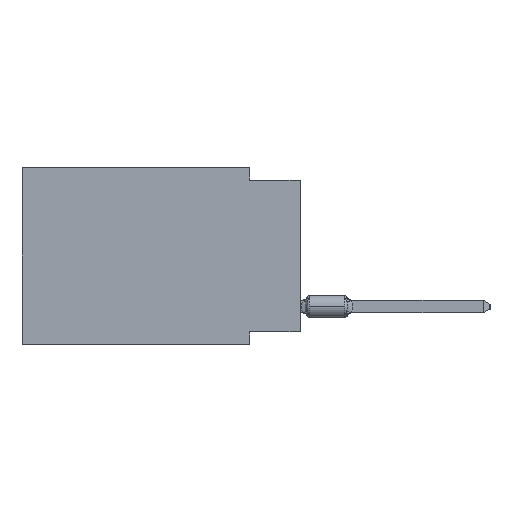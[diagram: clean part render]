
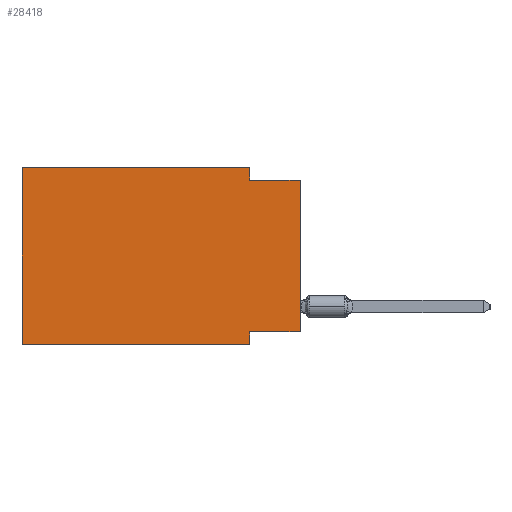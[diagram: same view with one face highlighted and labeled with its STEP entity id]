
A CAD part, left-side view. The second image highlights one B-rep face of the part: STEP entity #28418.
In plain terms, the highlighted planar face has unit normal (-1, 0, 0).
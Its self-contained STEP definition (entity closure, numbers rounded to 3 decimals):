
#78 = CARTESIAN_POINT ( 'NONE',  ( 0., 13.97, 0. ) ) ;
#1889 = AXIS2_PLACEMENT_3D ( 'NONE', #78, #43040, #19236 ) ;
#2113 = VECTOR ( 'NONE', #18753, 1000. ) ;
#2957 = VERTEX_POINT ( 'NONE', #48315 ) ;
#3211 = EDGE_CURVE ( 'NONE', #7900, #13524, #11572, .T. ) ;
#4538 = CARTESIAN_POINT ( 'NONE',  ( 0., 2.54, -8.89 ) ) ;
#5136 = DIRECTION ( 'NONE',  ( 0., 1., 0. ) ) ;
#5771 = CARTESIAN_POINT ( 'NONE',  ( 0., 2.54, -8.255 ) ) ;
#7900 = VERTEX_POINT ( 'NONE', #25880 ) ;
#8570 = ORIENTED_EDGE ( 'NONE', *, *, #16201, .F. ) ;
#8651 = VECTOR ( 'NONE', #5136, 1000. ) ;
#9314 = ORIENTED_EDGE ( 'NONE', *, *, #20235, .F. ) ;
#9891 = CARTESIAN_POINT ( 'NONE',  ( 0., 0., -0.635 ) ) ;
#10210 = ORIENTED_EDGE ( 'NONE', *, *, #34375, .F. ) ;
#11032 = ORIENTED_EDGE ( 'NONE', *, *, #39177, .T. ) ;
#11249 = CARTESIAN_POINT ( 'NONE',  ( 0., 2.54, 0. ) ) ;
#11399 = CARTESIAN_POINT ( 'NONE',  ( 0., 0., -8.255 ) ) ;
#11572 = LINE ( 'NONE', #50357, #26445 ) ;
#12261 = CARTESIAN_POINT ( 'NONE',  ( 0., 0., 0. ) ) ;
#12337 = CARTESIAN_POINT ( 'NONE',  ( 0., 0., -0.635 ) ) ;
#12630 = LINE ( 'NONE', #17725, #8651 ) ;
#13524 = VERTEX_POINT ( 'NONE', #48796 ) ;
#16201 = EDGE_CURVE ( 'NONE', #2957, #43560, #32501, .T. ) ;
#16347 = EDGE_LOOP ( 'NONE', ( #11032, #8570, #10210, #18486, #47995, #33762, #50886, #9314 ) ) ;
#16496 = VECTOR ( 'NONE', #38810, 1000. ) ;
#17725 = CARTESIAN_POINT ( 'NONE',  ( 0., 0., -8.255 ) ) ;
#18370 = VERTEX_POINT ( 'NONE', #31610 ) ;
#18486 = ORIENTED_EDGE ( 'NONE', *, *, #3211, .F. ) ;
#18753 = DIRECTION ( 'NONE',  ( 0., 0., -1. ) ) ;
#19012 = LINE ( 'NONE', #11249, #2113 ) ;
#19236 = DIRECTION ( 'NONE',  ( 0., 0., -1. ) ) ;
#20235 = EDGE_CURVE ( 'NONE', #24567, #39274, #12630, .T. ) ;
#22193 = LINE ( 'NONE', #26597, #25947 ) ;
#23030 = CARTESIAN_POINT ( 'NONE',  ( 0., 13.97, -8.89 ) ) ;
#23282 = LINE ( 'NONE', #23030, #16496 ) ;
#24567 = VERTEX_POINT ( 'NONE', #11399 ) ;
#25880 = CARTESIAN_POINT ( 'NONE',  ( 0., 13.97, 0. ) ) ;
#25947 = VECTOR ( 'NONE', #30477, 1000. ) ;
#26445 = VECTOR ( 'NONE', #42351, 1000. ) ;
#26597 = CARTESIAN_POINT ( 'NONE',  ( 0., 13.97, 0. ) ) ;
#27790 = LINE ( 'NONE', #12261, #35009 ) ;
#28418 = ADVANCED_FACE ( 'NONE', ( #39403 ), #35522, .F. ) ;
#28884 = DIRECTION ( 'NONE',  ( 0., -1., 0. ) ) ;
#30477 = DIRECTION ( 'NONE',  ( 0., 0., 1. ) ) ;
#31610 = CARTESIAN_POINT ( 'NONE',  ( 0., 2.54, -8.89 ) ) ;
#31718 = LINE ( 'NONE', #4538, #48836 ) ;
#32501 = LINE ( 'NONE', #12337, #37005 ) ;
#33762 = ORIENTED_EDGE ( 'NONE', *, *, #47013, .T. ) ;
#34375 = EDGE_CURVE ( 'NONE', #13524, #2957, #19012, .T. ) ;
#35009 = VECTOR ( 'NONE', #43568, 1000. ) ;
#35522 = PLANE ( 'NONE',  #1889 ) ;
#37005 = VECTOR ( 'NONE', #28884, 1000. ) ;
#38810 = DIRECTION ( 'NONE',  ( 0., -1., 0. ) ) ;
#39177 = EDGE_CURVE ( 'NONE', #24567, #43560, #27790, .T. ) ;
#39274 = VERTEX_POINT ( 'NONE', #5771 ) ;
#39403 = FACE_OUTER_BOUND ( 'NONE', #16347, .T. ) ;
#39718 = EDGE_CURVE ( 'NONE', #50684, #7900, #22193, .T. ) ;
#42351 = DIRECTION ( 'NONE',  ( 0., -1., 0. ) ) ;
#43040 = DIRECTION ( 'NONE',  ( 1., 0., 0. ) ) ;
#43560 = VERTEX_POINT ( 'NONE', #9891 ) ;
#43568 = DIRECTION ( 'NONE',  ( 0., 0., 1. ) ) ;
#43875 = DIRECTION ( 'NONE',  ( 0., 0., -1. ) ) ;
#46036 = CARTESIAN_POINT ( 'NONE',  ( 0., 13.97, -8.89 ) ) ;
#47013 = EDGE_CURVE ( 'NONE', #50684, #18370, #23282, .T. ) ;
#47995 = ORIENTED_EDGE ( 'NONE', *, *, #39718, .F. ) ;
#48315 = CARTESIAN_POINT ( 'NONE',  ( 0., 2.54, -0.635 ) ) ;
#48796 = CARTESIAN_POINT ( 'NONE',  ( 0., 2.54, 0. ) ) ;
#48836 = VECTOR ( 'NONE', #43875, 1000. ) ;
#50088 = EDGE_CURVE ( 'NONE', #39274, #18370, #31718, .T. ) ;
#50357 = CARTESIAN_POINT ( 'NONE',  ( 0., 13.97, 0. ) ) ;
#50684 = VERTEX_POINT ( 'NONE', #46036 ) ;
#50886 = ORIENTED_EDGE ( 'NONE', *, *, #50088, .F. ) ;
